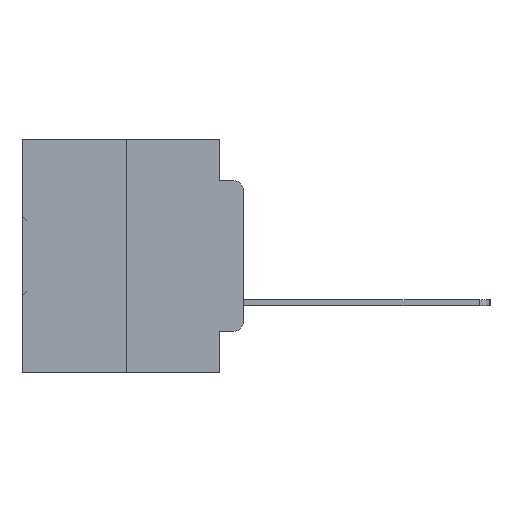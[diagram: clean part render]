
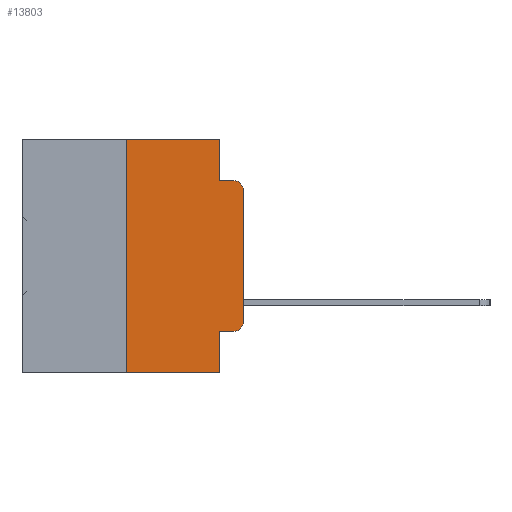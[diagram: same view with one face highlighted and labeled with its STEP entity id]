
A CAD part, left-side view. The second image highlights one B-rep face of the part: STEP entity #13803.
In plain terms, the highlighted planar face has unit normal (-1, 0, 0).
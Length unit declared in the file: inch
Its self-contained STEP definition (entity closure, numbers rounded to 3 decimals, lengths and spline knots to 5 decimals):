
#106 = DIRECTION ( 'NONE',  ( 1., 0., 0. ) ) ;
#1055 = CARTESIAN_POINT ( 'NONE',  ( 0., 0., -0.3915 ) ) ;
#2008 = VERTEX_POINT ( 'NONE', #23088 ) ;
#2288 = DIRECTION ( 'NONE',  ( 0., 0., -1. ) ) ;
#3280 = CIRCLE ( 'NONE', #28194, 0.02 ) ;
#3570 = VERTEX_POINT ( 'NONE', #12597 ) ;
#3874 = EDGE_CURVE ( 'NONE', #34436, #21682, #6253, .T. ) ;
#5361 = LINE ( 'NONE', #8051, #33777 ) ;
#5612 = CARTESIAN_POINT ( 'NONE',  ( 0., 0.25, 0. ) ) ;
#6253 = LINE ( 'NONE', #5612, #27380 ) ;
#7101 = DIRECTION ( 'NONE',  ( 0., -1., 0. ) ) ;
#7190 = LINE ( 'NONE', #13531, #21094 ) ;
#7644 = EDGE_CURVE ( 'NONE', #2008, #3570, #3280, .T. ) ;
#7806 = ORIENTED_EDGE ( 'NONE', *, *, #28121, .F. ) ;
#7938 = CARTESIAN_POINT ( 'NONE',  ( 0., 0.02, -0.1085 ) ) ;
#7989 = LINE ( 'NONE', #32669, #14492 ) ;
#8051 = CARTESIAN_POINT ( 'NONE',  ( 0., 0.473, -0.5 ) ) ;
#9507 = EDGE_CURVE ( 'NONE', #24326, #3570, #7989, .T. ) ;
#9655 = LINE ( 'NONE', #15367, #17044 ) ;
#10245 = CARTESIAN_POINT ( 'NONE',  ( 0., 0.051, -0.5 ) ) ;
#10714 = DIRECTION ( 'NONE',  ( 0., 0., -1. ) ) ;
#10839 = DIRECTION ( 'NONE',  ( 0., -1., 0. ) ) ;
#11556 = EDGE_CURVE ( 'NONE', #28210, #12245, #13530, .T. ) ;
#11797 = CARTESIAN_POINT ( 'NONE',  ( 0., 0., 0. ) ) ;
#11986 = DIRECTION ( 'NONE',  ( -1., 0., 0. ) ) ;
#12245 = VERTEX_POINT ( 'NONE', #1055 ) ;
#12484 = VECTOR ( 'NONE', #14593, 39.37008 ) ;
#12568 = CARTESIAN_POINT ( 'NONE',  ( 0., 0.051, -0.4115 ) ) ;
#12597 = CARTESIAN_POINT ( 'NONE',  ( 0., 0.02, -0.0885 ) ) ;
#13359 = LINE ( 'NONE', #11797, #12484 ) ;
#13530 = CIRCLE ( 'NONE', #35608, 0.02 ) ;
#13531 = CARTESIAN_POINT ( 'NONE',  ( 0., 0.051, 0. ) ) ;
#13552 = CARTESIAN_POINT ( 'NONE',  ( 0., 0.25, 0. ) ) ;
#13803 = ADVANCED_FACE ( 'NONE', ( #15603 ), #33178, .F. ) ;
#14492 = VECTOR ( 'NONE', #35389, 39.37008 ) ;
#14593 = DIRECTION ( 'NONE',  ( 0., 0., 1. ) ) ;
#15315 = DIRECTION ( 'NONE',  ( 0., 0., -1. ) ) ;
#15367 = CARTESIAN_POINT ( 'NONE',  ( 0., 0.473, 0. ) ) ;
#15532 = AXIS2_PLACEMENT_3D ( 'NONE', #24979, #106, #19635 ) ;
#15603 = FACE_OUTER_BOUND ( 'NONE', #35663, .T. ) ;
#17044 = VECTOR ( 'NONE', #34473, 39.37008 ) ;
#17696 = DIRECTION ( 'NONE',  ( 0., 0., 1. ) ) ;
#18369 = EDGE_CURVE ( 'NONE', #21682, #23921, #9655, .T. ) ;
#18670 = ORIENTED_EDGE ( 'NONE', *, *, #34545, .T. ) ;
#19542 = ORIENTED_EDGE ( 'NONE', *, *, #24513, .T. ) ;
#19635 = DIRECTION ( 'NONE',  ( 0., 0., -1. ) ) ;
#19961 = ORIENTED_EDGE ( 'NONE', *, *, #7644, .T. ) ;
#20322 = VERTEX_POINT ( 'NONE', #10245 ) ;
#20605 = CARTESIAN_POINT ( 'NONE',  ( 0., 0.051, 0. ) ) ;
#20662 = EDGE_CURVE ( 'NONE', #12245, #2008, #13359, .T. ) ;
#21094 = VECTOR ( 'NONE', #2288, 39.37008 ) ;
#21381 = CARTESIAN_POINT ( 'NONE',  ( 0., 0.25, -0.5 ) ) ;
#21682 = VERTEX_POINT ( 'NONE', #13552 ) ;
#22681 = EDGE_CURVE ( 'NONE', #24479, #20322, #32060, .T. ) ;
#23088 = CARTESIAN_POINT ( 'NONE',  ( 0., 0., -0.1085 ) ) ;
#23377 = ORIENTED_EDGE ( 'NONE', *, *, #18369, .F. ) ;
#23501 = CARTESIAN_POINT ( 'NONE',  ( 0., 0.051, 0. ) ) ;
#23921 = VERTEX_POINT ( 'NONE', #20605 ) ;
#24230 = ORIENTED_EDGE ( 'NONE', *, *, #3874, .F. ) ;
#24326 = VERTEX_POINT ( 'NONE', #28288 ) ;
#24479 = VERTEX_POINT ( 'NONE', #12568 ) ;
#24513 = EDGE_CURVE ( 'NONE', #24479, #28210, #34036, .T. ) ;
#24979 = CARTESIAN_POINT ( 'NONE',  ( 0., 0.473, 0. ) ) ;
#25675 = VECTOR ( 'NONE', #15315, 39.37008 ) ;
#27166 = DIRECTION ( 'NONE',  ( -1., 0., 0. ) ) ;
#27380 = VECTOR ( 'NONE', #17696, 39.37008 ) ;
#27540 = CARTESIAN_POINT ( 'NONE',  ( 0., 0.02, -0.4115 ) ) ;
#28121 = EDGE_CURVE ( 'NONE', #23921, #24326, #7190, .T. ) ;
#28194 = AXIS2_PLACEMENT_3D ( 'NONE', #7938, #27166, #10714 ) ;
#28210 = VERTEX_POINT ( 'NONE', #27540 ) ;
#28288 = CARTESIAN_POINT ( 'NONE',  ( 0., 0.051, -0.0885 ) ) ;
#28427 = CARTESIAN_POINT ( 'NONE',  ( 0., 0.02, -0.3915 ) ) ;
#28876 = ORIENTED_EDGE ( 'NONE', *, *, #9507, .F. ) ;
#31166 = DIRECTION ( 'NONE',  ( 0., 0., -1. ) ) ;
#32060 = LINE ( 'NONE', #23501, #25675 ) ;
#32352 = VECTOR ( 'NONE', #7101, 39.37008 ) ;
#32669 = CARTESIAN_POINT ( 'NONE',  ( 0., 0.051, -0.0885 ) ) ;
#33158 = ORIENTED_EDGE ( 'NONE', *, *, #22681, .F. ) ;
#33178 = PLANE ( 'NONE',  #15532 ) ;
#33550 = ORIENTED_EDGE ( 'NONE', *, *, #20662, .T. ) ;
#33777 = VECTOR ( 'NONE', #10839, 39.37008 ) ;
#34036 = LINE ( 'NONE', #34474, #32352 ) ;
#34436 = VERTEX_POINT ( 'NONE', #21381 ) ;
#34473 = DIRECTION ( 'NONE',  ( 0., -1., 0. ) ) ;
#34474 = CARTESIAN_POINT ( 'NONE',  ( 0., 0.051, -0.4115 ) ) ;
#34545 = EDGE_CURVE ( 'NONE', #34436, #20322, #5361, .T. ) ;
#35389 = DIRECTION ( 'NONE',  ( 0., -1., 0. ) ) ;
#35608 = AXIS2_PLACEMENT_3D ( 'NONE', #28427, #11986, #31166 ) ;
#35663 = EDGE_LOOP ( 'NONE', ( #33550, #19961, #28876, #7806, #23377, #24230, #18670, #33158, #19542, #35705 ) ) ;
#35705 = ORIENTED_EDGE ( 'NONE', *, *, #11556, .T. ) ;
